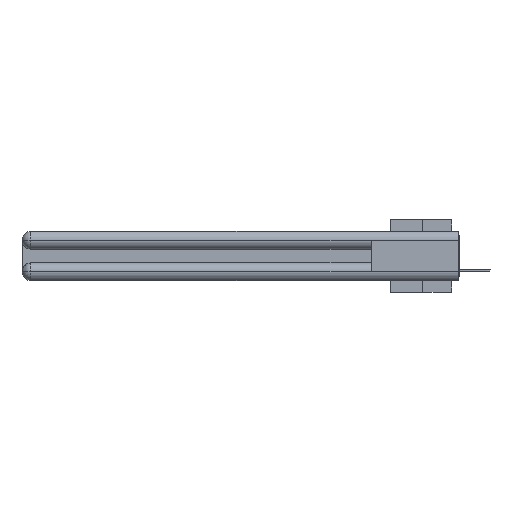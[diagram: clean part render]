
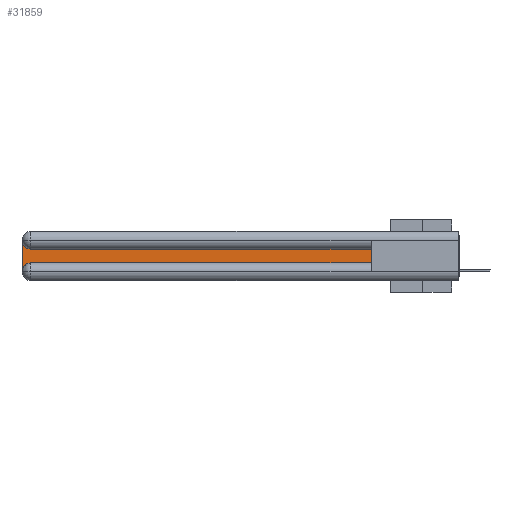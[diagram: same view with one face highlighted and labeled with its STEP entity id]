
A CAD part, left-side view. The second image highlights one B-rep face of the part: STEP entity #31859.
In plain terms, the highlighted planar face has unit normal (-1, 0, 0).
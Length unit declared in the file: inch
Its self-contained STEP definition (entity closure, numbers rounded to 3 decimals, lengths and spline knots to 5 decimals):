
#164 = ORIENTED_EDGE ( 'NONE', *, *, #32450, .T. ) ;
#1969 = LINE ( 'NONE', #21591, #32534 ) ;
#2114 = ORIENTED_EDGE ( 'NONE', *, *, #6683, .T. ) ;
#2663 = AXIS2_PLACEMENT_3D ( 'NONE', #16218, #7909, #5258 ) ;
#3946 = CARTESIAN_POINT ( 'NONE',  ( 0.075, 3., -0.0625 ) ) ;
#4045 = CARTESIAN_POINT ( 'NONE',  ( 0.075, 0.6, -0.2175 ) ) ;
#5258 = DIRECTION ( 'NONE',  ( 0., 0., -1. ) ) ;
#5608 = EDGE_CURVE ( 'NONE', #29236, #35115, #10219, .T. ) ;
#6683 = EDGE_CURVE ( 'NONE', #9422, #7285, #26033, .T. ) ;
#7285 = VERTEX_POINT ( 'NONE', #35014 ) ;
#7345 = LINE ( 'NONE', #20607, #24159 ) ;
#7558 = CARTESIAN_POINT ( 'NONE',  ( 0.075, 3., -0.2775 ) ) ;
#7909 = DIRECTION ( 'NONE',  ( 1., 0., 0. ) ) ;
#8785 = LINE ( 'NONE', #32949, #35045 ) ;
#9141 = ORIENTED_EDGE ( 'NONE', *, *, #13802, .T. ) ;
#9422 = VERTEX_POINT ( 'NONE', #7558 ) ;
#10219 = LINE ( 'NONE', #32644, #13189 ) ;
#11192 = CARTESIAN_POINT ( 'NONE',  ( 0.075, 2.94, -0.2775 ) ) ;
#12495 = DIRECTION ( 'NONE',  ( 0., -1., 0. ) ) ;
#13189 = VECTOR ( 'NONE', #18967, 39.37008 ) ;
#13802 = EDGE_CURVE ( 'NONE', #34143, #9422, #8785, .T. ) ;
#14580 = ORIENTED_EDGE ( 'NONE', *, *, #17602, .T. ) ;
#15818 = FACE_OUTER_BOUND ( 'NONE', #23724, .T. ) ;
#16218 = CARTESIAN_POINT ( 'NONE',  ( 0.075, 3., -0.1225 ) ) ;
#16765 = ORIENTED_EDGE ( 'NONE', *, *, #5608, .T. ) ;
#17602 = EDGE_CURVE ( 'NONE', #7285, #18115, #7345, .T. ) ;
#17874 = AXIS2_PLACEMENT_3D ( 'NONE', #18598, #32279, #26887 ) ;
#18115 = VERTEX_POINT ( 'NONE', #4045 ) ;
#18598 = CARTESIAN_POINT ( 'NONE',  ( 0.075, 2.94, -0.0625 ) ) ;
#18967 = DIRECTION ( 'NONE',  ( 0., 1., 0. ) ) ;
#19237 = DIRECTION ( 'NONE',  ( 1., 0., 0. ) ) ;
#20607 = CARTESIAN_POINT ( 'NONE',  ( 0.075, 0.6, -0.2175 ) ) ;
#20987 = EDGE_CURVE ( 'NONE', #18115, #29236, #1969, .T. ) ;
#21591 = CARTESIAN_POINT ( 'NONE',  ( 0.075, 0.6, -0.2175 ) ) ;
#22395 = CARTESIAN_POINT ( 'NONE',  ( 0.075, 0.6, -0.1225 ) ) ;
#23724 = EDGE_LOOP ( 'NONE', ( #16765, #164, #9141, #2114, #14580, #25258 ) ) ;
#24159 = VECTOR ( 'NONE', #12495, 39.37008 ) ;
#24402 = PLANE ( 'NONE',  #2663 ) ;
#25258 = ORIENTED_EDGE ( 'NONE', *, *, #20987, .T. ) ;
#26033 = CIRCLE ( 'NONE', #35657, 0.06 ) ;
#26887 = DIRECTION ( 'NONE',  ( 0., 0., -1. ) ) ;
#29236 = VERTEX_POINT ( 'NONE', #22395 ) ;
#29319 = DIRECTION ( 'NONE',  ( 0., 0., -1. ) ) ;
#31859 = ADVANCED_FACE ( 'NONE', ( #15818 ), #24402, .F. ) ;
#32279 = DIRECTION ( 'NONE',  ( 1., 0., 0. ) ) ;
#32450 = EDGE_CURVE ( 'NONE', #35115, #34143, #34659, .T. ) ;
#32507 = DIRECTION ( 'NONE',  ( 0., 0., 1. ) ) ;
#32534 = VECTOR ( 'NONE', #32507, 39.37008 ) ;
#32644 = CARTESIAN_POINT ( 'NONE',  ( 0.075, 0.6, -0.1225 ) ) ;
#32949 = CARTESIAN_POINT ( 'NONE',  ( 0.075, 3., -0.2175 ) ) ;
#34143 = VERTEX_POINT ( 'NONE', #3946 ) ;
#34659 = CIRCLE ( 'NONE', #17874, 0.06 ) ;
#34746 = DIRECTION ( 'NONE',  ( 0., 0., -1. ) ) ;
#35014 = CARTESIAN_POINT ( 'NONE',  ( 0.075, 2.94, -0.2175 ) ) ;
#35045 = VECTOR ( 'NONE', #34746, 39.37008 ) ;
#35115 = VERTEX_POINT ( 'NONE', #35187 ) ;
#35187 = CARTESIAN_POINT ( 'NONE',  ( 0.075, 2.94, -0.1225 ) ) ;
#35657 = AXIS2_PLACEMENT_3D ( 'NONE', #11192, #19237, #29319 ) ;
